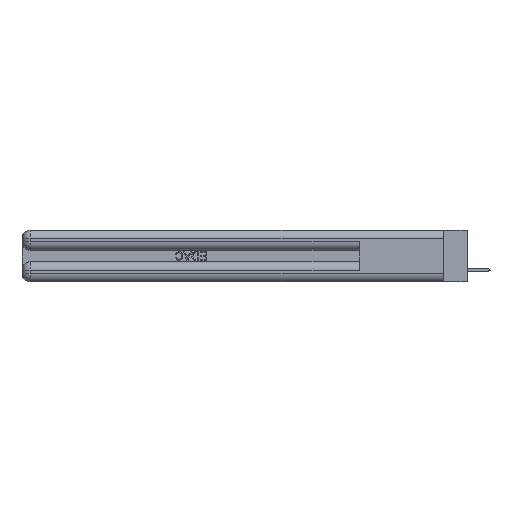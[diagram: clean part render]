
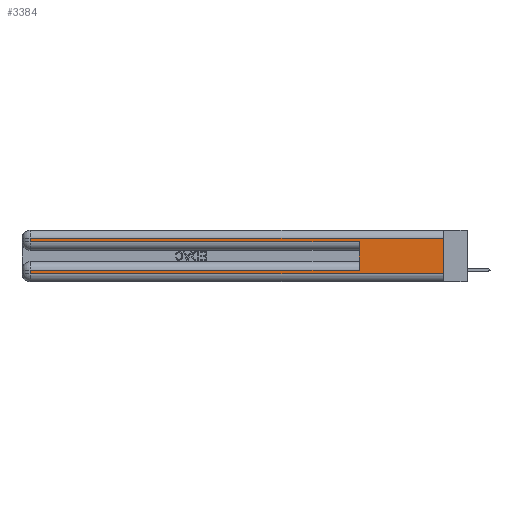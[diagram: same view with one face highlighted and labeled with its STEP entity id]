
A CAD part, left-side view. The second image highlights one B-rep face of the part: STEP entity #3384.
In plain terms, the highlighted planar face has unit normal (-1, 0, 0).
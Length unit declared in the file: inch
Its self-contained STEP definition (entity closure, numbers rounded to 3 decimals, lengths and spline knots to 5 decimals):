
#162 = LINE ( 'NONE', #35737, #9447 ) ;
#931 = PLANE ( 'NONE',  #14589 ) ;
#1075 = CARTESIAN_POINT ( 'NONE',  ( 0., 0., 0.37 ) ) ;
#1164 = LINE ( 'NONE', #35678, #31444 ) ;
#1416 = CARTESIAN_POINT ( 'NONE',  ( 0., 2.94, 0.06 ) ) ;
#3384 = ADVANCED_FACE ( 'NONE', ( #42071 ), #931, .F. ) ;
#3709 = DIRECTION ( 'NONE',  ( 0., 0., 1. ) ) ;
#3743 = VECTOR ( 'NONE', #28700, 39.37008 ) ;
#6514 = DIRECTION ( 'NONE',  ( 0., 0., -1. ) ) ;
#7209 = VERTEX_POINT ( 'NONE', #28373 ) ;
#9447 = VECTOR ( 'NONE', #39724, 39.37008 ) ;
#9793 = EDGE_CURVE ( 'NONE', #7209, #12840, #50678, .T. ) ;
#10770 = CARTESIAN_POINT ( 'NONE',  ( 0., 2.94, 0.285 ) ) ;
#10945 = ORIENTED_EDGE ( 'NONE', *, *, #36282, .F. ) ;
#11360 = CARTESIAN_POINT ( 'NONE',  ( 0., 2.94, 0.31 ) ) ;
#11544 = EDGE_CURVE ( 'NONE', #11742, #30251, #35639, .T. ) ;
#11742 = VERTEX_POINT ( 'NONE', #1416 ) ;
#12831 = CARTESIAN_POINT ( 'NONE',  ( 0., 0., 0.37 ) ) ;
#12840 = VERTEX_POINT ( 'NONE', #36212 ) ;
#13004 = DIRECTION ( 'NONE',  ( 1., 0., 0. ) ) ;
#14589 = AXIS2_PLACEMENT_3D ( 'NONE', #12831, #13004, #28379 ) ;
#15908 = CARTESIAN_POINT ( 'NONE',  ( 0., 0.6, 0.285 ) ) ;
#17462 = VERTEX_POINT ( 'NONE', #15908 ) ;
#17897 = VECTOR ( 'NONE', #37825, 39.37008 ) ;
#18518 = EDGE_CURVE ( 'NONE', #43110, #32578, #44929, .T. ) ;
#18957 = VECTOR ( 'NONE', #28244, 39.37008 ) ;
#19882 = ORIENTED_EDGE ( 'NONE', *, *, #18518, .T. ) ;
#21606 = CARTESIAN_POINT ( 'NONE',  ( 0., 0., 0.31 ) ) ;
#22411 = LINE ( 'NONE', #37603, #46482 ) ;
#22578 = VECTOR ( 'NONE', #23178, 39.37008 ) ;
#23178 = DIRECTION ( 'NONE',  ( 0., 0., -1. ) ) ;
#24317 = CARTESIAN_POINT ( 'NONE',  ( 0., 0., 0.06 ) ) ;
#24711 = CARTESIAN_POINT ( 'NONE',  ( 0., 0., 0.085 ) ) ;
#26082 = VERTEX_POINT ( 'NONE', #10770 ) ;
#26175 = ORIENTED_EDGE ( 'NONE', *, *, #11544, .T. ) ;
#27513 = CARTESIAN_POINT ( 'NONE',  ( 0., 0., 0.31 ) ) ;
#28216 = ORIENTED_EDGE ( 'NONE', *, *, #9793, .T. ) ;
#28244 = DIRECTION ( 'NONE',  ( 0., -1., 0. ) ) ;
#28373 = CARTESIAN_POINT ( 'NONE',  ( 0., 0.6, 0.085 ) ) ;
#28379 = DIRECTION ( 'NONE',  ( 0., 0., -1. ) ) ;
#28700 = DIRECTION ( 'NONE',  ( 0., 0., -1. ) ) ;
#29193 = ORIENTED_EDGE ( 'NONE', *, *, #29325, .T. ) ;
#29325 = EDGE_CURVE ( 'NONE', #32578, #26082, #31792, .T. ) ;
#30251 = VERTEX_POINT ( 'NONE', #44742 ) ;
#30445 = CARTESIAN_POINT ( 'NONE',  ( 0., 2.94, 0.37 ) ) ;
#30555 = EDGE_CURVE ( 'NONE', #26082, #17462, #162, .T. ) ;
#30952 = LINE ( 'NONE', #1075, #3743 ) ;
#31444 = VECTOR ( 'NONE', #3709, 39.37008 ) ;
#31582 = ORIENTED_EDGE ( 'NONE', *, *, #34796, .T. ) ;
#31792 = LINE ( 'NONE', #30445, #22578 ) ;
#32578 = VERTEX_POINT ( 'NONE', #11360 ) ;
#34460 = VECTOR ( 'NONE', #37317, 39.37008 ) ;
#34796 = EDGE_CURVE ( 'NONE', #12840, #11742, #22411, .T. ) ;
#35639 = LINE ( 'NONE', #24317, #18957 ) ;
#35678 = CARTESIAN_POINT ( 'NONE',  ( 0., 0.6, 0.145 ) ) ;
#35737 = CARTESIAN_POINT ( 'NONE',  ( 0., 0., 0.285 ) ) ;
#36212 = CARTESIAN_POINT ( 'NONE',  ( 0., 2.94, 0.085 ) ) ;
#36282 = EDGE_CURVE ( 'NONE', #7209, #17462, #1164, .T. ) ;
#36436 = ORIENTED_EDGE ( 'NONE', *, *, #30555, .T. ) ;
#37317 = DIRECTION ( 'NONE',  ( 0., 1., 0. ) ) ;
#37603 = CARTESIAN_POINT ( 'NONE',  ( 0., 2.94, 0.37 ) ) ;
#37825 = DIRECTION ( 'NONE',  ( 0., 1., 0. ) ) ;
#39514 = EDGE_LOOP ( 'NONE', ( #50380, #19882, #29193, #36436, #10945, #28216, #31582, #26175 ) ) ;
#39724 = DIRECTION ( 'NONE',  ( 0., -1., 0. ) ) ;
#42071 = FACE_OUTER_BOUND ( 'NONE', #39514, .T. ) ;
#43110 = VERTEX_POINT ( 'NONE', #27513 ) ;
#44742 = CARTESIAN_POINT ( 'NONE',  ( 0., 0., 0.06 ) ) ;
#44929 = LINE ( 'NONE', #21606, #34460 ) ;
#46482 = VECTOR ( 'NONE', #6514, 39.37008 ) ;
#47414 = EDGE_CURVE ( 'NONE', #43110, #30251, #30952, .T. ) ;
#50380 = ORIENTED_EDGE ( 'NONE', *, *, #47414, .F. ) ;
#50678 = LINE ( 'NONE', #24711, #17897 ) ;
